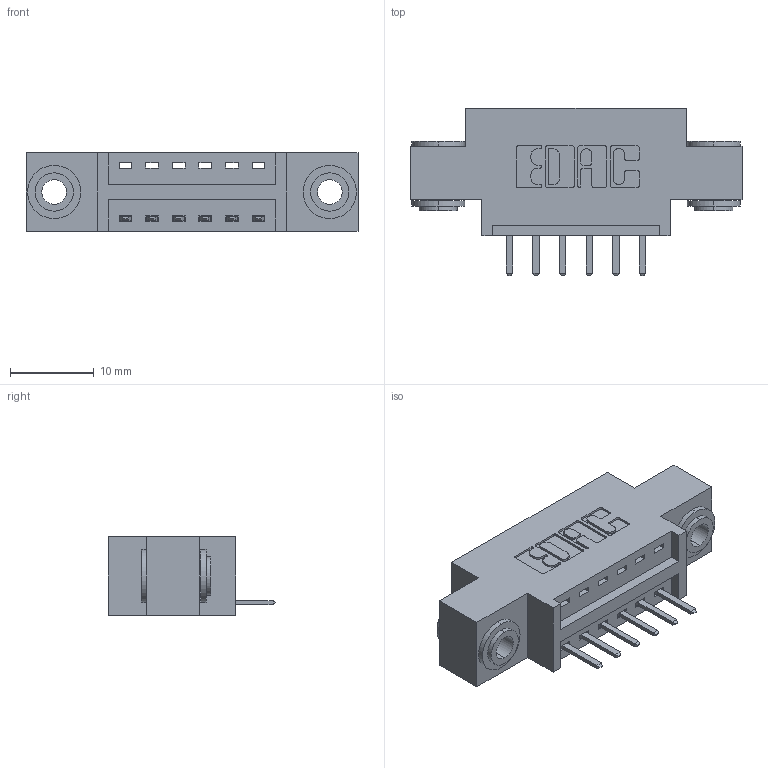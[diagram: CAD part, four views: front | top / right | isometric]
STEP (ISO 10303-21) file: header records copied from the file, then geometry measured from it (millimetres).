
FILE_DESCRIPTION (( 'STEP AP203' ), '1' );
FILE_NAME ('396-006-520-603.STEP', '2018-08-30T22:38:26', ( '' ), ( '' ), 'SwSTEP 2.0', 'SolidWorks 2016', '' );
FILE_SCHEMA (( 'CONFIG_CONTROL_DESIGN' ));
Length unit declared in the file: inch
Products named in the file (4): 345-292-001_345-293-120; 345-250-002_345-250-002-102; 396-006-520-603; 346 Part_0.170 Offset - 0.156 Dia-TH
Assembly tree (9 placements, depth 2):
  396-006-520-603
    346 Part_0.170 Offset - 0.156 Dia-TH
    345-292-001_345-293-120  x6
    345-250-002_345-250-002-102  x2
Bounding box: 39.62 x 20.02 x 9.4 mm (x, y, z)
Volume: 3392.4 mm3; surface area: 4173.5 mm2
Topology: 9 solids, 9 shells, 536 faces, 1521 edges, 994 vertices
Faces by surface type: plane 342, cylinder 186, cone 8
Entity records: 9466 total; most frequent: CARTESIAN_POINT 1625, ORIENTED_EDGE 1546, DIRECTION 1495, EDGE_CURVE 773, LINE 589, VECTOR 589, VERTEX_POINT 510, AXIS2_PLACEMENT_3D 453
